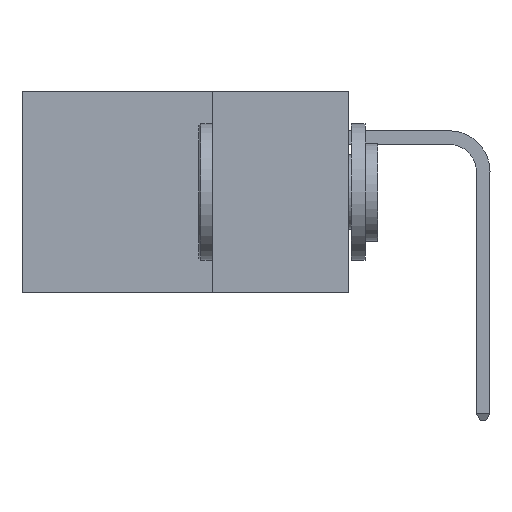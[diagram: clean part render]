
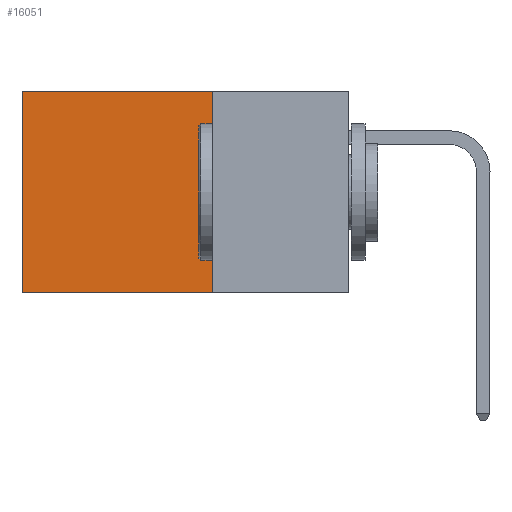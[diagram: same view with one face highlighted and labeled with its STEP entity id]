
A CAD part, left-side view. The second image highlights one B-rep face of the part: STEP entity #16051.
In plain terms, the highlighted planar face has unit normal (-1, 0, 0).
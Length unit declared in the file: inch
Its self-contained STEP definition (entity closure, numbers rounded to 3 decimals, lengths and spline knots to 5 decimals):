
#81 = CARTESIAN_POINT ( 'NONE',  ( 0.2875, 0.6, -0.37 ) ) ;
#1121 = EDGE_LOOP ( 'NONE', ( #32442, #23926, #32160, #24428 ) ) ;
#1374 = CARTESIAN_POINT ( 'NONE',  ( 0.2875, 0.6, 0. ) ) ;
#1664 = FACE_OUTER_BOUND ( 'NONE', #1121, .T. ) ;
#2537 = LINE ( 'NONE', #1374, #17906 ) ;
#2740 = CARTESIAN_POINT ( 'NONE',  ( 0.2875, 0.6, 0. ) ) ;
#3986 = AXIS2_PLACEMENT_3D ( 'NONE', #32470, #15769, #35236 ) ;
#4975 = CARTESIAN_POINT ( 'NONE',  ( 0.2875, 0.25, 0. ) ) ;
#5184 = CARTESIAN_POINT ( 'NONE',  ( 0.2875, 0.25, 0. ) ) ;
#7857 = LINE ( 'NONE', #11206, #22078 ) ;
#10003 = PLANE ( 'NONE',  #3986 ) ;
#10993 = CARTESIAN_POINT ( 'NONE',  ( 0.2875, 0.25, -0.37 ) ) ;
#11206 = CARTESIAN_POINT ( 'NONE',  ( 0.2875, 0.25, 0. ) ) ;
#11468 = VECTOR ( 'NONE', #36151, 39.37008 ) ;
#14767 = VERTEX_POINT ( 'NONE', #81 ) ;
#15769 = DIRECTION ( 'NONE',  ( 1., 0., 0. ) ) ;
#15876 = DIRECTION ( 'NONE',  ( 0., 0., -1. ) ) ;
#16051 = ADVANCED_FACE ( 'NONE', ( #1664 ), #10003, .F. ) ;
#17906 = VECTOR ( 'NONE', #15876, 39.37008 ) ;
#18615 = LINE ( 'NONE', #4975, #33433 ) ;
#19729 = DIRECTION ( 'NONE',  ( 0., 1., 0. ) ) ;
#22078 = VECTOR ( 'NONE', #19729, 39.37008 ) ;
#23926 = ORIENTED_EDGE ( 'NONE', *, *, #33557, .F. ) ;
#24206 = EDGE_CURVE ( 'NONE', #31701, #14767, #2537, .T. ) ;
#24428 = ORIENTED_EDGE ( 'NONE', *, *, #27025, .T. ) ;
#24862 = DIRECTION ( 'NONE',  ( 0., 0., -1. ) ) ;
#26293 = EDGE_CURVE ( 'NONE', #26969, #34757, #18615, .T. ) ;
#26969 = VERTEX_POINT ( 'NONE', #5184 ) ;
#27025 = EDGE_CURVE ( 'NONE', #26969, #31701, #7857, .T. ) ;
#31701 = VERTEX_POINT ( 'NONE', #2740 ) ;
#32160 = ORIENTED_EDGE ( 'NONE', *, *, #26293, .F. ) ;
#32442 = ORIENTED_EDGE ( 'NONE', *, *, #24206, .T. ) ;
#32470 = CARTESIAN_POINT ( 'NONE',  ( 0.2875, 0.25, 0. ) ) ;
#33370 = CARTESIAN_POINT ( 'NONE',  ( 0.2875, 0.25, -0.37 ) ) ;
#33433 = VECTOR ( 'NONE', #24862, 39.37008 ) ;
#33557 = EDGE_CURVE ( 'NONE', #34757, #14767, #33809, .T. ) ;
#33809 = LINE ( 'NONE', #33370, #11468 ) ;
#34757 = VERTEX_POINT ( 'NONE', #10993 ) ;
#35236 = DIRECTION ( 'NONE',  ( 0., 0., -1. ) ) ;
#36151 = DIRECTION ( 'NONE',  ( 0., 1., 0. ) ) ;
